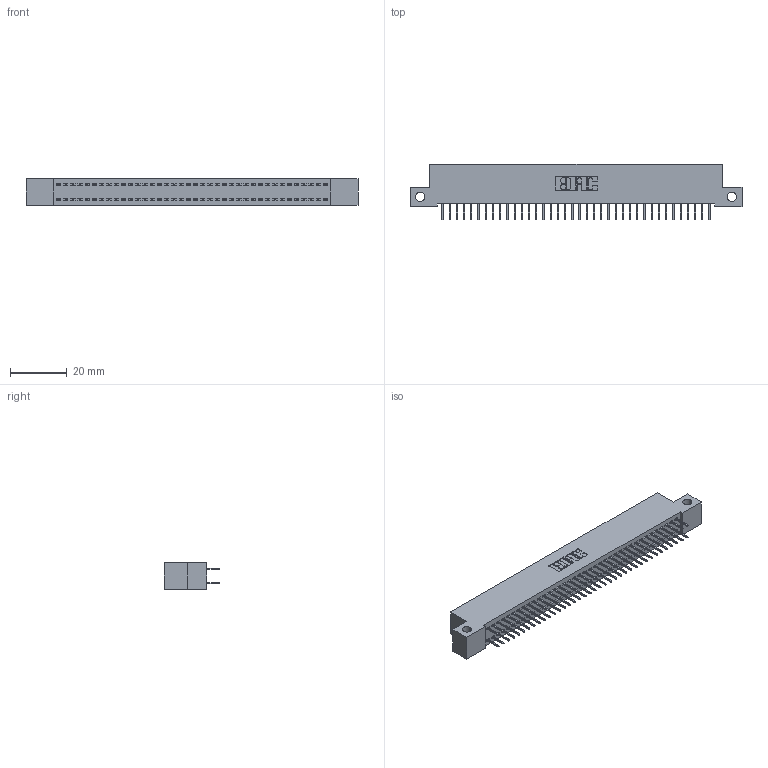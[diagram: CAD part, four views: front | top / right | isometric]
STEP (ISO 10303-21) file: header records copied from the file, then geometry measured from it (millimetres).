
FILE_DESCRIPTION (( 'STEP AP203' ), '1' );
FILE_NAME ('392-076-524-212.STEP', '2019-10-09T13:27:18', ( '' ), ( '' ), 'SwSTEP 2.0', 'SolidWorks 2016', '' );
FILE_SCHEMA (( 'CONFIG_CONTROL_DESIGN' ));
Length unit declared in the file: inch
Products named in the file (3): 342 Part_Side Mount; 345-292-001_345-293-124; 392-076-524-212
Assembly tree (77 placements, depth 2):
  392-076-524-212
    342 Part_Side Mount
    345-292-001_345-293-124  x76
Bounding box: 116.84 x 19.69 x 9.4 mm (x, y, z)
Volume: 10290.2 mm3; surface area: 16192.3 mm2
Topology: 77 solids, 77 shells, 4366 faces, 12383 edges, 7950 vertices
Faces by surface type: plane 3258, cylinder 1108
Entity records: 24909 total; most frequent: CARTESIAN_POINT 4130, ORIENTED_EDGE 4066, DIRECTION 3537, EDGE_CURVE 2033, VECTOR 1909, LINE 1909, VERTEX_POINT 1350, AXIS2_PLACEMENT_3D 814
